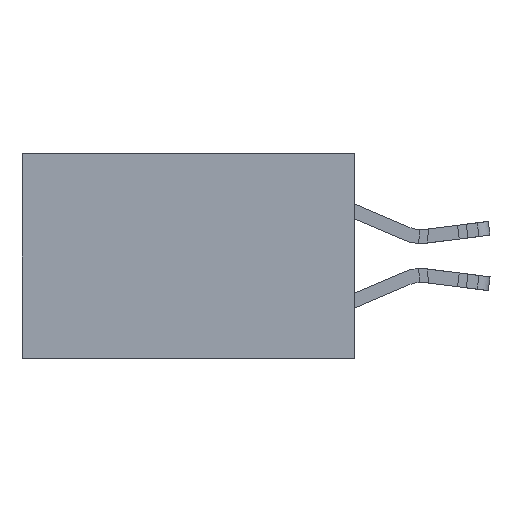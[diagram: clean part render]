
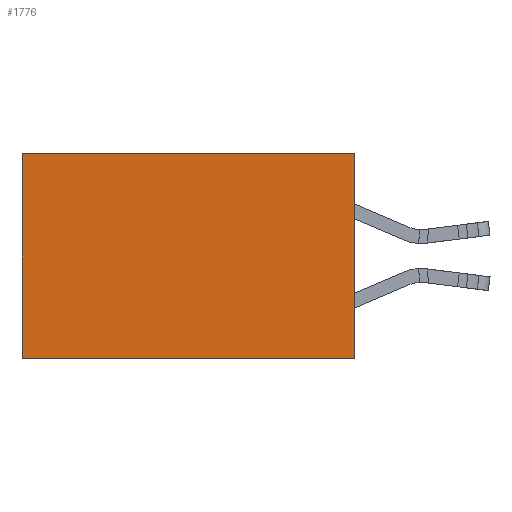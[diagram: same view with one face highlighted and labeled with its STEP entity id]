
A CAD part, left-side view. The second image highlights one B-rep face of the part: STEP entity #1776.
In plain terms, the highlighted planar face has unit normal (-1, 0, 0).
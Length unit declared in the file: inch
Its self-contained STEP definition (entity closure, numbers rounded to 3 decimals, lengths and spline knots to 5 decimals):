
#777 = VECTOR ( 'NONE', #19709, 39.37008 ) ;
#1459 = LINE ( 'NONE', #4864, #777 ) ;
#1776 = ADVANCED_FACE ( 'NONE', ( #2488 ), #3966, .F. ) ;
#1850 = ORIENTED_EDGE ( 'NONE', *, *, #23111, .T. ) ;
#2488 = FACE_OUTER_BOUND ( 'NONE', #2986, .T. ) ;
#2986 = EDGE_LOOP ( 'NONE', ( #4988, #27555, #5532, #1850 ) ) ;
#3043 = LINE ( 'NONE', #13799, #8101 ) ;
#3146 = DIRECTION ( 'NONE',  ( 0., 0., -1. ) ) ;
#3625 = VERTEX_POINT ( 'NONE', #27455 ) ;
#3759 = LINE ( 'NONE', #22641, #10131 ) ;
#3956 = CARTESIAN_POINT ( 'NONE',  ( 0.2615, 0., -0.37 ) ) ;
#3966 = PLANE ( 'NONE',  #11338 ) ;
#4340 = DIRECTION ( 'NONE',  ( 0., 0., -1. ) ) ;
#4405 = VERTEX_POINT ( 'NONE', #17055 ) ;
#4864 = CARTESIAN_POINT ( 'NONE',  ( 0.2615, 0., -0.37 ) ) ;
#4988 = ORIENTED_EDGE ( 'NONE', *, *, #22685, .T. ) ;
#4990 = DIRECTION ( 'NONE',  ( 0., 0., -1. ) ) ;
#5385 = DIRECTION ( 'NONE',  ( 1., 0., 0. ) ) ;
#5532 = ORIENTED_EDGE ( 'NONE', *, *, #15190, .F. ) ;
#6520 = CARTESIAN_POINT ( 'NONE',  ( 0.2615, 0.6, -0.37 ) ) ;
#7805 = DIRECTION ( 'NONE',  ( 0., 1., 0. ) ) ;
#8101 = VECTOR ( 'NONE', #3146, 39.37008 ) ;
#8160 = VECTOR ( 'NONE', #4340, 39.37008 ) ;
#10131 = VECTOR ( 'NONE', #7805, 39.37008 ) ;
#11338 = AXIS2_PLACEMENT_3D ( 'NONE', #3956, #5385, #4990 ) ;
#13799 = CARTESIAN_POINT ( 'NONE',  ( 0.2615, 0., -0.37 ) ) ;
#15190 = EDGE_CURVE ( 'NONE', #3625, #19742, #3043, .T. ) ;
#17055 = CARTESIAN_POINT ( 'NONE',  ( 0.2615, 0.6, -0.37 ) ) ;
#18101 = CARTESIAN_POINT ( 'NONE',  ( 0.2615, 0., -0.37 ) ) ;
#19709 = DIRECTION ( 'NONE',  ( 0., 1., 0. ) ) ;
#19742 = VERTEX_POINT ( 'NONE', #18101 ) ;
#21577 = EDGE_CURVE ( 'NONE', #19742, #4405, #1459, .T. ) ;
#22641 = CARTESIAN_POINT ( 'NONE',  ( 0.2615, 0., 0. ) ) ;
#22685 = EDGE_CURVE ( 'NONE', #25247, #4405, #24486, .T. ) ;
#23111 = EDGE_CURVE ( 'NONE', #3625, #25247, #3759, .T. ) ;
#24486 = LINE ( 'NONE', #6520, #8160 ) ;
#25247 = VERTEX_POINT ( 'NONE', #25345 ) ;
#25345 = CARTESIAN_POINT ( 'NONE',  ( 0.2615, 0.6, 0. ) ) ;
#27455 = CARTESIAN_POINT ( 'NONE',  ( 0.2615, 0., 0. ) ) ;
#27555 = ORIENTED_EDGE ( 'NONE', *, *, #21577, .F. ) ;
